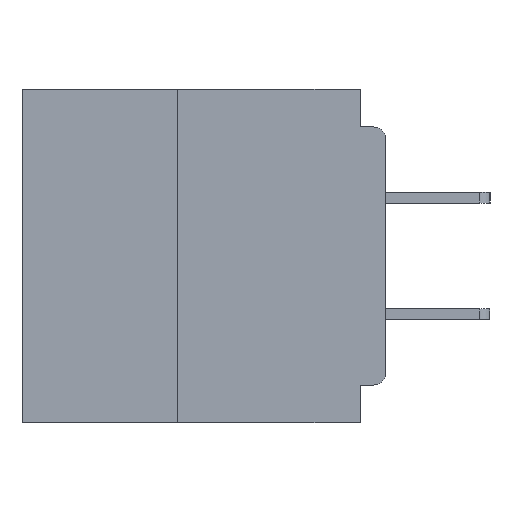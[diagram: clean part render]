
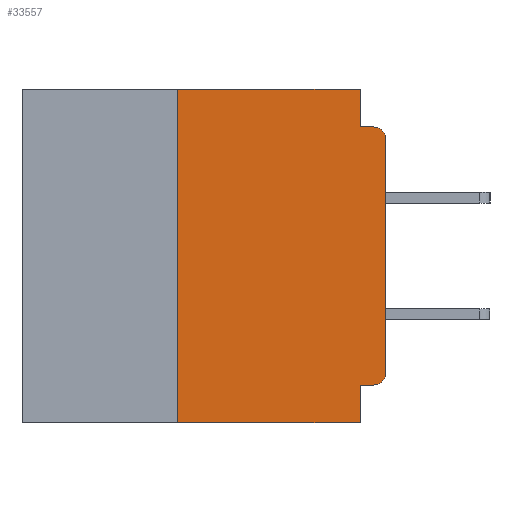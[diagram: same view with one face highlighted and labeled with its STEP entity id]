
A CAD part, left-side view. The second image highlights one B-rep face of the part: STEP entity #33557.
In plain terms, the highlighted planar face has unit normal (-1, 0, 0).
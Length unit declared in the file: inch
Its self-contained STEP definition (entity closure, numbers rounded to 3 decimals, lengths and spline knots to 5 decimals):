
#154 = VERTEX_POINT ( 'NONE', #5681 ) ;
#350 = EDGE_CURVE ( 'NONE', #3009, #28245, #19172, .T. ) ;
#1634 = ORIENTED_EDGE ( 'NONE', *, *, #10282, .F. ) ;
#2629 = VERTEX_POINT ( 'NONE', #10172 ) ;
#3009 = VERTEX_POINT ( 'NONE', #34308 ) ;
#3174 = CARTESIAN_POINT ( 'NONE',  ( 0., 0.015, -0.06 ) ) ;
#3681 = EDGE_CURVE ( 'NONE', #154, #6015, #7642, .T. ) ;
#4331 = CARTESIAN_POINT ( 'NONE',  ( 0., 0.437, 0. ) ) ;
#4476 = DIRECTION ( 'NONE',  ( 1., 0., 0. ) ) ;
#5320 = LINE ( 'NONE', #32699, #6312 ) ;
#5681 = CARTESIAN_POINT ( 'NONE',  ( 0., 0., -0.06 ) ) ;
#5876 = AXIS2_PLACEMENT_3D ( 'NONE', #4331, #4476, #26857 ) ;
#6015 = VERTEX_POINT ( 'NONE', #13691 ) ;
#6312 = VECTOR ( 'NONE', #13716, 39.37008 ) ;
#6406 = DIRECTION ( 'NONE',  ( 0., 0., -1. ) ) ;
#6880 = CARTESIAN_POINT ( 'NONE',  ( 0., 0.25, -0.4 ) ) ;
#7380 = ORIENTED_EDGE ( 'NONE', *, *, #350, .F. ) ;
#7642 = CIRCLE ( 'NONE', #25812, 0.015 ) ;
#8231 = DIRECTION ( 'NONE',  ( 0., 1., 0. ) ) ;
#9480 = CARTESIAN_POINT ( 'NONE',  ( 0., 0.031, -0.4 ) ) ;
#10172 = CARTESIAN_POINT ( 'NONE',  ( 0., 0.015, -0.355 ) ) ;
#10282 = EDGE_CURVE ( 'NONE', #2629, #38906, #29025, .T. ) ;
#10599 = VECTOR ( 'NONE', #30183, 39.37008 ) ;
#10822 = PLANE ( 'NONE',  #5876 ) ;
#12021 = FACE_OUTER_BOUND ( 'NONE', #29698, .T. ) ;
#12685 = DIRECTION ( 'NONE',  ( 0., 0., -1. ) ) ;
#13649 = CARTESIAN_POINT ( 'NONE',  ( 0., 0.015, -0.34 ) ) ;
#13691 = CARTESIAN_POINT ( 'NONE',  ( 0., 0.015, -0.045 ) ) ;
#13716 = DIRECTION ( 'NONE',  ( 0., -1., 0. ) ) ;
#14018 = VERTEX_POINT ( 'NONE', #16636 ) ;
#15001 = VECTOR ( 'NONE', #12685, 39.37008 ) ;
#15851 = DIRECTION ( 'NONE',  ( 0., 0., -1. ) ) ;
#16134 = CARTESIAN_POINT ( 'NONE',  ( 0., 0.25, 0. ) ) ;
#16545 = LINE ( 'NONE', #37953, #39733 ) ;
#16636 = CARTESIAN_POINT ( 'NONE',  ( 0., 0.031, 0. ) ) ;
#16900 = DIRECTION ( 'NONE',  ( 0., 0., -1. ) ) ;
#17382 = ORIENTED_EDGE ( 'NONE', *, *, #3681, .T. ) ;
#18186 = EDGE_CURVE ( 'NONE', #38906, #24421, #23484, .T. ) ;
#19073 = EDGE_CURVE ( 'NONE', #3009, #24421, #5320, .T. ) ;
#19172 = LINE ( 'NONE', #6880, #10599 ) ;
#19296 = VECTOR ( 'NONE', #29470, 39.37008 ) ;
#19354 = DIRECTION ( 'NONE',  ( 0., -1., 0. ) ) ;
#19423 = ORIENTED_EDGE ( 'NONE', *, *, #20828, .F. ) ;
#20331 = LINE ( 'NONE', #26282, #19296 ) ;
#20756 = LINE ( 'NONE', #36075, #37414 ) ;
#20828 = EDGE_CURVE ( 'NONE', #14018, #37963, #16545, .T. ) ;
#21665 = EDGE_CURVE ( 'NONE', #2629, #38867, #40638, .T. ) ;
#22893 = LINE ( 'NONE', #35052, #38599 ) ;
#23198 = EDGE_CURVE ( 'NONE', #37963, #6015, #22893, .T. ) ;
#23434 = DIRECTION ( 'NONE',  ( 0., -1., 0. ) ) ;
#23470 = AXIS2_PLACEMENT_3D ( 'NONE', #13649, #35811, #16900 ) ;
#23484 = LINE ( 'NONE', #9480, #15001 ) ;
#23801 = ORIENTED_EDGE ( 'NONE', *, *, #18186, .F. ) ;
#24026 = ORIENTED_EDGE ( 'NONE', *, *, #19073, .T. ) ;
#24392 = EDGE_CURVE ( 'NONE', #38867, #154, #20331, .T. ) ;
#24421 = VERTEX_POINT ( 'NONE', #26417 ) ;
#25394 = EDGE_CURVE ( 'NONE', #28245, #14018, #20756, .T. ) ;
#25591 = DIRECTION ( 'NONE',  ( -1., 0., 0. ) ) ;
#25812 = AXIS2_PLACEMENT_3D ( 'NONE', #3174, #25591, #6406 ) ;
#26282 = CARTESIAN_POINT ( 'NONE',  ( 0., 0., 0. ) ) ;
#26394 = CARTESIAN_POINT ( 'NONE',  ( 0., 0.031, -0.045 ) ) ;
#26417 = CARTESIAN_POINT ( 'NONE',  ( 0., 0.031, -0.4 ) ) ;
#26706 = ORIENTED_EDGE ( 'NONE', *, *, #25394, .F. ) ;
#26857 = DIRECTION ( 'NONE',  ( 0., 0., -1. ) ) ;
#28245 = VERTEX_POINT ( 'NONE', #16134 ) ;
#29025 = LINE ( 'NONE', #36716, #36386 ) ;
#29437 = ORIENTED_EDGE ( 'NONE', *, *, #24392, .T. ) ;
#29470 = DIRECTION ( 'NONE',  ( 0., 0., 1. ) ) ;
#29698 = EDGE_LOOP ( 'NONE', ( #29437, #17382, #30912, #19423, #26706, #7380, #24026, #23801, #1634, #37093 ) ) ;
#30183 = DIRECTION ( 'NONE',  ( 0., 0., 1. ) ) ;
#30912 = ORIENTED_EDGE ( 'NONE', *, *, #23198, .F. ) ;
#32699 = CARTESIAN_POINT ( 'NONE',  ( 0., 0.437, -0.4 ) ) ;
#33557 = ADVANCED_FACE ( 'NONE', ( #12021 ), #10822, .F. ) ;
#34093 = CARTESIAN_POINT ( 'NONE',  ( 0., 0.031, -0.355 ) ) ;
#34308 = CARTESIAN_POINT ( 'NONE',  ( 0., 0.25, -0.4 ) ) ;
#35052 = CARTESIAN_POINT ( 'NONE',  ( 0., 0., -0.045 ) ) ;
#35811 = DIRECTION ( 'NONE',  ( -1., 0., 0. ) ) ;
#36075 = CARTESIAN_POINT ( 'NONE',  ( 0., 0.437, 0. ) ) ;
#36386 = VECTOR ( 'NONE', #8231, 39.37008 ) ;
#36716 = CARTESIAN_POINT ( 'NONE',  ( 0., 0., -0.355 ) ) ;
#36978 = CARTESIAN_POINT ( 'NONE',  ( 0., 0., -0.34 ) ) ;
#37093 = ORIENTED_EDGE ( 'NONE', *, *, #21665, .T. ) ;
#37414 = VECTOR ( 'NONE', #23434, 39.37008 ) ;
#37953 = CARTESIAN_POINT ( 'NONE',  ( 0., 0.031, 0. ) ) ;
#37963 = VERTEX_POINT ( 'NONE', #26394 ) ;
#38599 = VECTOR ( 'NONE', #19354, 39.37008 ) ;
#38867 = VERTEX_POINT ( 'NONE', #36978 ) ;
#38906 = VERTEX_POINT ( 'NONE', #34093 ) ;
#39733 = VECTOR ( 'NONE', #15851, 39.37008 ) ;
#40638 = CIRCLE ( 'NONE', #23470, 0.015 ) ;
